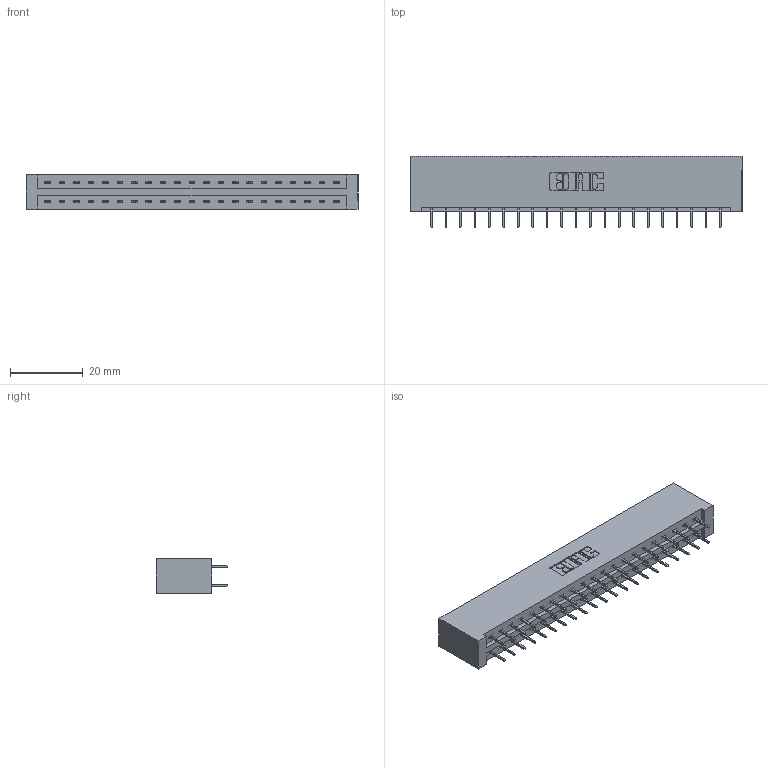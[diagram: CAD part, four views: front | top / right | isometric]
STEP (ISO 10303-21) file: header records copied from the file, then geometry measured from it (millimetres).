
FILE_DESCRIPTION (( 'STEP AP203' ), '1' );
FILE_NAME ('337-042-524-201.STEP', '2018-08-08T23:46:19', ( '' ), ( '' ), 'SwSTEP 2.0', 'SolidWorks 2016', '' );
FILE_SCHEMA (( 'CONFIG_CONTROL_DESIGN' ));
Length unit declared in the file: inch
Products named in the file (3): 337 Part_No Mounting Lugs; 345-292-001_345-293-124; 337-042-524-201
Assembly tree (43 placements, depth 2):
  337-042-524-201
    337 Part_No Mounting Lugs
    345-292-001_345-293-124  x42
Bounding box: 91.08 x 19.69 x 9.4 mm (x, y, z)
Volume: 10016.8 mm3; surface area: 10979.3 mm2
Topology: 43 solids, 43 shells, 2542 faces, 7217 edges, 4642 vertices
Faces by surface type: plane 1914, cylinder 628
Entity records: 18795 total; most frequent: CARTESIAN_POINT 3182, ORIENTED_EDGE 3118, DIRECTION 2739, EDGE_CURVE 1559, LINE 1443, VECTOR 1443, VERTEX_POINT 1034, AXIS2_PLACEMENT_3D 648
